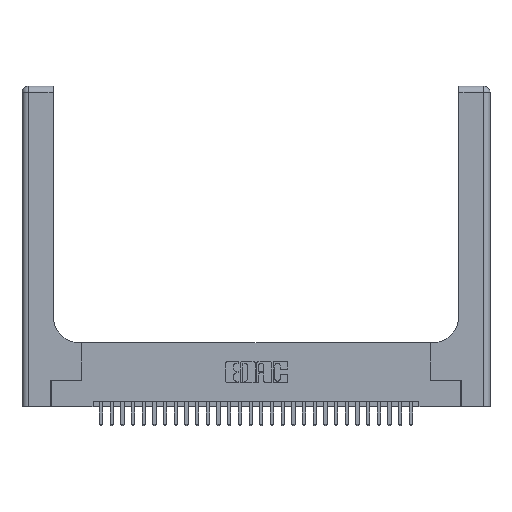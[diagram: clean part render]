
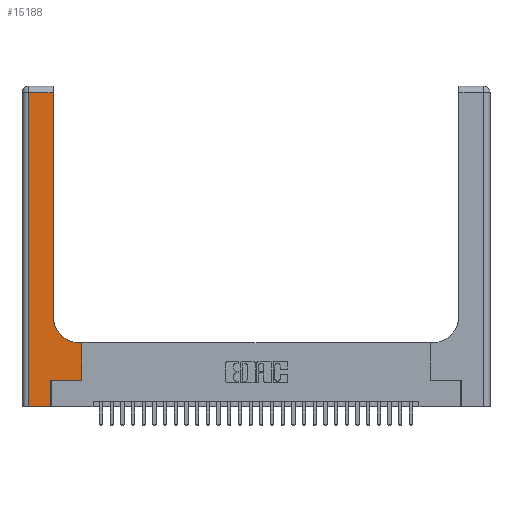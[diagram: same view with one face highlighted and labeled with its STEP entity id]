
A CAD part, top view. The second image highlights one B-rep face of the part: STEP entity #15188.
In plain terms, the highlighted planar face has unit normal (0, 0, 1).
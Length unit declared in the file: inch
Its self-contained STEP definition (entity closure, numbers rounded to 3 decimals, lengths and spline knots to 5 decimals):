
#307 = DIRECTION ( 'NONE',  ( 0., -1., 0. ) ) ;
#372 = VECTOR ( 'NONE', #19680, 39.37008 ) ;
#730 = EDGE_CURVE ( 'NONE', #6109, #1845, #12952, .T. ) ;
#848 = ORIENTED_EDGE ( 'NONE', *, *, #12652, .T. ) ;
#1442 = ORIENTED_EDGE ( 'NONE', *, *, #2387, .T. ) ;
#1845 = VERTEX_POINT ( 'NONE', #19032 ) ;
#2202 = LINE ( 'NONE', #2675, #25884 ) ;
#2237 = EDGE_CURVE ( 'NONE', #8046, #12995, #5914, .T. ) ;
#2292 = VECTOR ( 'NONE', #22659, 39.37008 ) ;
#2387 = EDGE_CURVE ( 'NONE', #4622, #17254, #2932, .T. ) ;
#2675 = CARTESIAN_POINT ( 'NONE',  ( 0.269, 0.25, 0.37 ) ) ;
#2708 = FACE_OUTER_BOUND ( 'NONE', #18839, .T. ) ;
#2794 = CARTESIAN_POINT ( 'NONE',  ( 0.2915, 3., 0.37 ) ) ;
#2932 = LINE ( 'NONE', #4276, #20290 ) ;
#3243 = VECTOR ( 'NONE', #4935, 39.37008 ) ;
#3990 = VECTOR ( 'NONE', #5202, 39.37008 ) ;
#4276 = CARTESIAN_POINT ( 'NONE',  ( 0.5585, 0.25, 0.37 ) ) ;
#4622 = VERTEX_POINT ( 'NONE', #13385 ) ;
#4904 = VERTEX_POINT ( 'NONE', #19497 ) ;
#4935 = DIRECTION ( 'NONE',  ( 1., 0., 0. ) ) ;
#5202 = DIRECTION ( 'NONE',  ( 0., 1., 0. ) ) ;
#5777 = EDGE_CURVE ( 'NONE', #17254, #8046, #8562, .T. ) ;
#5914 = CIRCLE ( 'NONE', #8030, 0.25 ) ;
#6109 = VERTEX_POINT ( 'NONE', #19025 ) ;
#6155 = CARTESIAN_POINT ( 'NONE',  ( 0.2915, 0.6, 0.37 ) ) ;
#6727 = VECTOR ( 'NONE', #19599, 39.37008 ) ;
#7017 = CARTESIAN_POINT ( 'NONE',  ( 0., 3., 0.37 ) ) ;
#8030 = AXIS2_PLACEMENT_3D ( 'NONE', #22754, #8566, #25117 ) ;
#8046 = VERTEX_POINT ( 'NONE', #21612 ) ;
#8562 = LINE ( 'NONE', #6155, #2292 ) ;
#8566 = DIRECTION ( 'NONE',  ( 0., 0., -1. ) ) ;
#8576 = CARTESIAN_POINT ( 'NONE',  ( 0.2915, 0.85, 0.37 ) ) ;
#8692 = EDGE_CURVE ( 'NONE', #12995, #4904, #10946, .T. ) ;
#9394 = DIRECTION ( 'NONE',  ( 0., 0., -1. ) ) ;
#10946 = LINE ( 'NONE', #2794, #3990 ) ;
#12454 = CARTESIAN_POINT ( 'NONE',  ( 0.269, 0., 0.37 ) ) ;
#12590 = EDGE_CURVE ( 'NONE', #27429, #6109, #27618, .T. ) ;
#12652 = EDGE_CURVE ( 'NONE', #21215, #27429, #14306, .T. ) ;
#12952 = LINE ( 'NONE', #12454, #6727 ) ;
#12995 = VERTEX_POINT ( 'NONE', #8576 ) ;
#13385 = CARTESIAN_POINT ( 'NONE',  ( 0.5585, 0.25, 0.37 ) ) ;
#14306 = LINE ( 'NONE', #28591, #19869 ) ;
#14335 = ORIENTED_EDGE ( 'NONE', *, *, #17920, .T. ) ;
#14683 = ORIENTED_EDGE ( 'NONE', *, *, #730, .T. ) ;
#15188 = ADVANCED_FACE ( 'NONE', ( #2708 ), #23583, .F. ) ;
#16628 = ORIENTED_EDGE ( 'NONE', *, *, #5777, .T. ) ;
#17254 = VERTEX_POINT ( 'NONE', #21994 ) ;
#17920 = EDGE_CURVE ( 'NONE', #1845, #4622, #2202, .T. ) ;
#18394 = DIRECTION ( 'NONE',  ( 0., 1., 0. ) ) ;
#18667 = ORIENTED_EDGE ( 'NONE', *, *, #2237, .T. ) ;
#18839 = EDGE_LOOP ( 'NONE', ( #20447, #25644, #848, #23806, #14683, #14335, #1442, #16628, #18667 ) ) ;
#19025 = CARTESIAN_POINT ( 'NONE',  ( 0.269, 0., 0.37 ) ) ;
#19032 = CARTESIAN_POINT ( 'NONE',  ( 0.269, 0.25, 0.37 ) ) ;
#19043 = CARTESIAN_POINT ( 'NONE',  ( 0., 0., 0.37 ) ) ;
#19497 = CARTESIAN_POINT ( 'NONE',  ( 0.2915, 2.94, 0.37 ) ) ;
#19599 = DIRECTION ( 'NONE',  ( 0., 1., 0. ) ) ;
#19680 = DIRECTION ( 'NONE',  ( -1., 0., 0. ) ) ;
#19869 = VECTOR ( 'NONE', #307, 39.37008 ) ;
#19979 = EDGE_CURVE ( 'NONE', #4904, #21215, #24821, .T. ) ;
#20290 = VECTOR ( 'NONE', #18394, 39.37008 ) ;
#20447 = ORIENTED_EDGE ( 'NONE', *, *, #8692, .T. ) ;
#20492 = CARTESIAN_POINT ( 'NONE',  ( 0.06, 2.94, 0.37 ) ) ;
#21215 = VERTEX_POINT ( 'NONE', #20492 ) ;
#21230 = CARTESIAN_POINT ( 'NONE',  ( 0.06, 0., 0.37 ) ) ;
#21571 = DIRECTION ( 'NONE',  ( 1., 0., 0. ) ) ;
#21612 = CARTESIAN_POINT ( 'NONE',  ( 0.5415, 0.6, 0.37 ) ) ;
#21994 = CARTESIAN_POINT ( 'NONE',  ( 0.5585, 0.6, 0.37 ) ) ;
#22584 = AXIS2_PLACEMENT_3D ( 'NONE', #7017, #9394, #25945 ) ;
#22659 = DIRECTION ( 'NONE',  ( -1., 0., 0. ) ) ;
#22754 = CARTESIAN_POINT ( 'NONE',  ( 0.5415, 0.85, 0.37 ) ) ;
#23583 = PLANE ( 'NONE',  #22584 ) ;
#23806 = ORIENTED_EDGE ( 'NONE', *, *, #12590, .T. ) ;
#24821 = LINE ( 'NONE', #29109, #372 ) ;
#25117 = DIRECTION ( 'NONE',  ( 1., 0., 0. ) ) ;
#25644 = ORIENTED_EDGE ( 'NONE', *, *, #19979, .T. ) ;
#25884 = VECTOR ( 'NONE', #21571, 39.37008 ) ;
#25945 = DIRECTION ( 'NONE',  ( -1., 0., 0. ) ) ;
#27429 = VERTEX_POINT ( 'NONE', #21230 ) ;
#27618 = LINE ( 'NONE', #19043, #3243 ) ;
#28591 = CARTESIAN_POINT ( 'NONE',  ( 0.06, 3., 0.37 ) ) ;
#29109 = CARTESIAN_POINT ( 'NONE',  ( 0., 2.94, 0.37 ) ) ;
